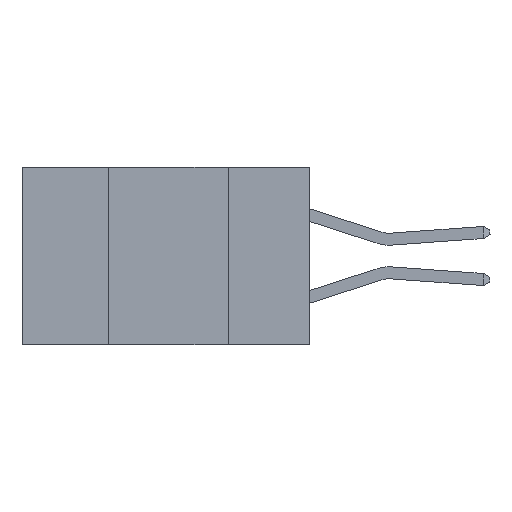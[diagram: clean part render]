
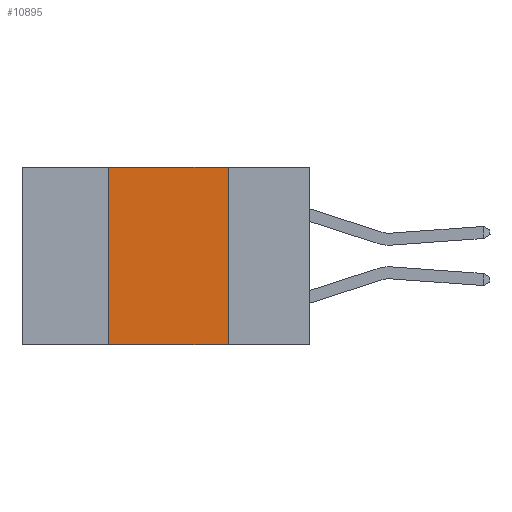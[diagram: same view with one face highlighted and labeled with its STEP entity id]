
A CAD part, left-side view. The second image highlights one B-rep face of the part: STEP entity #10895.
In plain terms, the highlighted planar face has unit normal (-1, 0, 0).
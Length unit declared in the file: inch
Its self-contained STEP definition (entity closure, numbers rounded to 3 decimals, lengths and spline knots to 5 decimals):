
#1023 = CARTESIAN_POINT ( 'NONE',  ( 0., 0.17, 0. ) ) ;
#1757 = CARTESIAN_POINT ( 'NONE',  ( 0., 0.6, -0.37 ) ) ;
#1978 = CARTESIAN_POINT ( 'NONE',  ( 0., 0.42, -0.37 ) ) ;
#2463 = CARTESIAN_POINT ( 'NONE',  ( 0., 0.42, 0. ) ) ;
#3809 = ORIENTED_EDGE ( 'NONE', *, *, #4185, .F. ) ;
#3902 = VERTEX_POINT ( 'NONE', #7347 ) ;
#4185 = EDGE_CURVE ( 'NONE', #18215, #6910, #4513, .T. ) ;
#4513 = LINE ( 'NONE', #25638, #11308 ) ;
#6169 = ORIENTED_EDGE ( 'NONE', *, *, #11954, .T. ) ;
#6637 = VECTOR ( 'NONE', #27135, 39.37008 ) ;
#6752 = VECTOR ( 'NONE', #10757, 39.37008 ) ;
#6910 = VERTEX_POINT ( 'NONE', #1023 ) ;
#7347 = CARTESIAN_POINT ( 'NONE',  ( 0., 0.42, -0.37 ) ) ;
#7996 = LINE ( 'NONE', #1757, #16374 ) ;
#8844 = EDGE_CURVE ( 'NONE', #3902, #18215, #21130, .T. ) ;
#10230 = EDGE_LOOP ( 'NONE', ( #18761, #3809, #13413, #6169 ) ) ;
#10757 = DIRECTION ( 'NONE',  ( 0., 0., -1. ) ) ;
#10895 = ADVANCED_FACE ( 'NONE', ( #23915 ), #25886, .F. ) ;
#11308 = VECTOR ( 'NONE', #26055, 39.37008 ) ;
#11954 = EDGE_CURVE ( 'NONE', #3902, #16957, #7996, .T. ) ;
#13236 = CARTESIAN_POINT ( 'NONE',  ( 0., 0.6, 0. ) ) ;
#13413 = ORIENTED_EDGE ( 'NONE', *, *, #8844, .F. ) ;
#16374 = VECTOR ( 'NONE', #26910, 39.37008 ) ;
#16957 = VERTEX_POINT ( 'NONE', #19265 ) ;
#18215 = VERTEX_POINT ( 'NONE', #2463 ) ;
#18761 = ORIENTED_EDGE ( 'NONE', *, *, #22309, .F. ) ;
#19265 = CARTESIAN_POINT ( 'NONE',  ( 0., 0.17, -0.37 ) ) ;
#20794 = AXIS2_PLACEMENT_3D ( 'NONE', #13236, #21709, #21565 ) ;
#21130 = LINE ( 'NONE', #1978, #6637 ) ;
#21565 = DIRECTION ( 'NONE',  ( 0., 0., -1. ) ) ;
#21709 = DIRECTION ( 'NONE',  ( 1., 0., 0. ) ) ;
#21717 = LINE ( 'NONE', #23250, #6752 ) ;
#22309 = EDGE_CURVE ( 'NONE', #6910, #16957, #21717, .T. ) ;
#23250 = CARTESIAN_POINT ( 'NONE',  ( 0., 0.17, -0.37 ) ) ;
#23915 = FACE_OUTER_BOUND ( 'NONE', #10230, .T. ) ;
#25638 = CARTESIAN_POINT ( 'NONE',  ( 0., 0.6, 0. ) ) ;
#25886 = PLANE ( 'NONE',  #20794 ) ;
#26055 = DIRECTION ( 'NONE',  ( 0., -1., 0. ) ) ;
#26910 = DIRECTION ( 'NONE',  ( 0., -1., 0. ) ) ;
#27135 = DIRECTION ( 'NONE',  ( 0., 0., 1. ) ) ;
